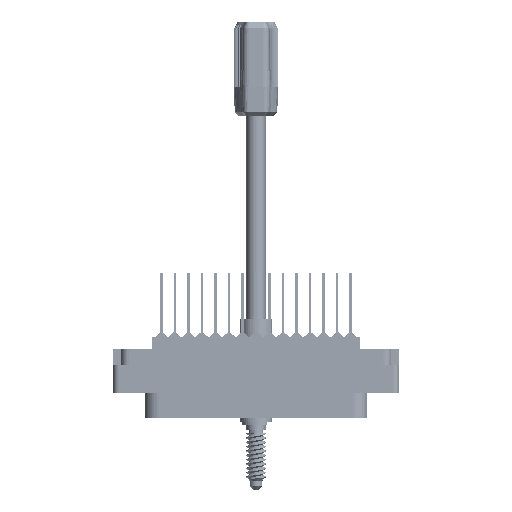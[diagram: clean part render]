
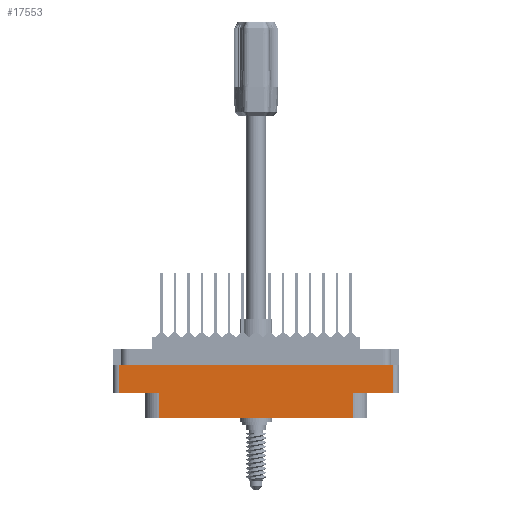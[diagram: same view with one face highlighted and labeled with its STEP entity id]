
A CAD part, front view. The second image highlights one B-rep face of the part: STEP entity #17553.
In plain terms, the highlighted planar face has unit normal (0, -1, 0).
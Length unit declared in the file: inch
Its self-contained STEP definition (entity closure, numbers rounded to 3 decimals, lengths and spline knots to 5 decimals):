
#322 = DIRECTION ( 'NONE',  ( 1., 0., 0. ) ) ;
#1789 = DIRECTION ( 'NONE',  ( 0., 0., -1. ) ) ;
#3356 = CARTESIAN_POINT ( 'NONE',  ( -0.9315, -0.7625, -0.54 ) ) ;
#3779 = LINE ( 'NONE', #45101, #36136 ) ;
#4277 = VERTEX_POINT ( 'NONE', #33186 ) ;
#5095 = DIRECTION ( 'NONE',  ( 0., 0., 1. ) ) ;
#5269 = DIRECTION ( 'NONE',  ( -1., 0., 0. ) ) ;
#6195 = VECTOR ( 'NONE', #57904, 39.37008 ) ;
#6654 = EDGE_CURVE ( 'NONE', #84105, #4277, #25009, .T. ) ;
#7618 = VECTOR ( 'NONE', #322, 39.37008 ) ;
#11736 = CARTESIAN_POINT ( 'NONE',  ( -1.313, -0.7625, -0.274 ) ) ;
#13922 = CARTESIAN_POINT ( 'NONE',  ( 0., -0.7625, -0.54 ) ) ;
#15768 = DIRECTION ( 'NONE',  ( 0., 0., 1. ) ) ;
#16184 = LINE ( 'NONE', #42481, #6195 ) ;
#17211 = VECTOR ( 'NONE', #5269, 39.37008 ) ;
#17553 = ADVANCED_FACE ( 'NONE', ( #88992 ), #73638, .T. ) ;
#19495 = EDGE_CURVE ( 'NONE', #28662, #43310, #16184, .T. ) ;
#20135 = LINE ( 'NONE', #95952, #7618 ) ;
#20317 = VECTOR ( 'NONE', #73661, 39.37008 ) ;
#20519 = VECTOR ( 'NONE', #75039, 39.37008 ) ;
#22849 = EDGE_CURVE ( 'NONE', #43310, #82765, #62908, .T. ) ;
#23046 = ORIENTED_EDGE ( 'NONE', *, *, #100842, .F. ) ;
#23428 = ORIENTED_EDGE ( 'NONE', *, *, #74686, .T. ) ;
#25009 = LINE ( 'NONE', #86308, #101310 ) ;
#28662 = VERTEX_POINT ( 'NONE', #11736 ) ;
#29002 = CARTESIAN_POINT ( 'NONE',  ( 1.313, -0.7625, -0.54 ) ) ;
#32874 = ORIENTED_EDGE ( 'NONE', *, *, #48412, .T. ) ;
#33186 = CARTESIAN_POINT ( 'NONE',  ( 0.9315, -0.7625, -0.54 ) ) ;
#33323 = ORIENTED_EDGE ( 'NONE', *, *, #96898, .F. ) ;
#33767 = CARTESIAN_POINT ( 'NONE',  ( -1.375, -0.7625, -0.78 ) ) ;
#36136 = VECTOR ( 'NONE', #5095, 39.37008 ) ;
#38113 = CARTESIAN_POINT ( 'NONE',  ( -0.9315, -0.7625, -0.78 ) ) ;
#41758 = ORIENTED_EDGE ( 'NONE', *, *, #22849, .T. ) ;
#42481 = CARTESIAN_POINT ( 'NONE',  ( -1.313, -0.7625, -0.78 ) ) ;
#43310 = VERTEX_POINT ( 'NONE', #99353 ) ;
#45050 = LINE ( 'NONE', #91554, #63810 ) ;
#45101 = CARTESIAN_POINT ( 'NONE',  ( 1.313, -0.7625, -0.78 ) ) ;
#46139 = ORIENTED_EDGE ( 'NONE', *, *, #6654, .T. ) ;
#47217 = CARTESIAN_POINT ( 'NONE',  ( 1.313, -0.7625, -0.274 ) ) ;
#48412 = EDGE_CURVE ( 'NONE', #82765, #74382, #77809, .T. ) ;
#49500 = DIRECTION ( 'NONE',  ( 0., -1., 0. ) ) ;
#50343 = VERTEX_POINT ( 'NONE', #29002 ) ;
#51167 = CARTESIAN_POINT ( 'NONE',  ( 0.9315, -0.7625, -0.78 ) ) ;
#51250 = AXIS2_PLACEMENT_3D ( 'NONE', #33767, #49500, #1789 ) ;
#57904 = DIRECTION ( 'NONE',  ( 0., 0., -1. ) ) ;
#57909 = CARTESIAN_POINT ( 'NONE',  ( -0.9315, -0.7625, -0.78 ) ) ;
#61436 = EDGE_CURVE ( 'NONE', #50343, #66282, #3779, .T. ) ;
#62908 = LINE ( 'NONE', #97459, #20519 ) ;
#63810 = VECTOR ( 'NONE', #75780, 39.37008 ) ;
#66282 = VERTEX_POINT ( 'NONE', #47217 ) ;
#73638 = PLANE ( 'NONE',  #51250 ) ;
#73661 = DIRECTION ( 'NONE',  ( 0., 0., -1. ) ) ;
#74382 = VERTEX_POINT ( 'NONE', #38113 ) ;
#74686 = EDGE_CURVE ( 'NONE', #74382, #84105, #45050, .T. ) ;
#75039 = DIRECTION ( 'NONE',  ( 1., 0., 0. ) ) ;
#75780 = DIRECTION ( 'NONE',  ( 1., 0., 0. ) ) ;
#77809 = LINE ( 'NONE', #57909, #20317 ) ;
#80892 = ORIENTED_EDGE ( 'NONE', *, *, #61436, .T. ) ;
#80937 = LINE ( 'NONE', #13922, #17211 ) ;
#82765 = VERTEX_POINT ( 'NONE', #3356 ) ;
#84105 = VERTEX_POINT ( 'NONE', #51167 ) ;
#86308 = CARTESIAN_POINT ( 'NONE',  ( 0.9315, -0.7625, -0.54 ) ) ;
#88992 = FACE_OUTER_BOUND ( 'NONE', #89499, .T. ) ;
#89499 = EDGE_LOOP ( 'NONE', ( #23046, #92019, #41758, #32874, #23428, #46139, #33323, #80892 ) ) ;
#91554 = CARTESIAN_POINT ( 'NONE',  ( -1.375, -0.7625, -0.78 ) ) ;
#92019 = ORIENTED_EDGE ( 'NONE', *, *, #19495, .T. ) ;
#95952 = CARTESIAN_POINT ( 'NONE',  ( 0., -0.7625, -0.274 ) ) ;
#96898 = EDGE_CURVE ( 'NONE', #50343, #4277, #80937, .T. ) ;
#97459 = CARTESIAN_POINT ( 'NONE',  ( 0., -0.7625, -0.54 ) ) ;
#99353 = CARTESIAN_POINT ( 'NONE',  ( -1.313, -0.7625, -0.54 ) ) ;
#100842 = EDGE_CURVE ( 'NONE', #28662, #66282, #20135, .T. ) ;
#101310 = VECTOR ( 'NONE', #15768, 39.37008 ) ;
